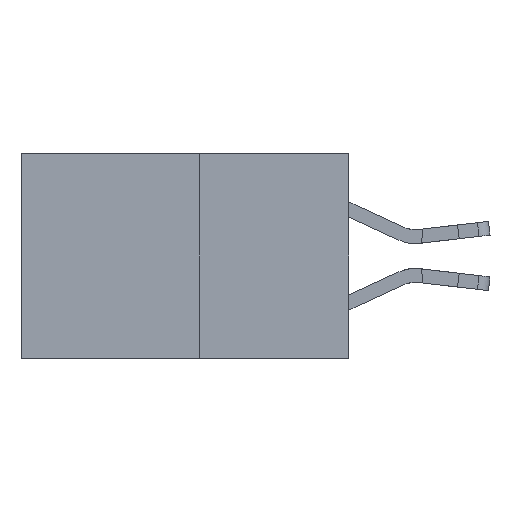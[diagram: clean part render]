
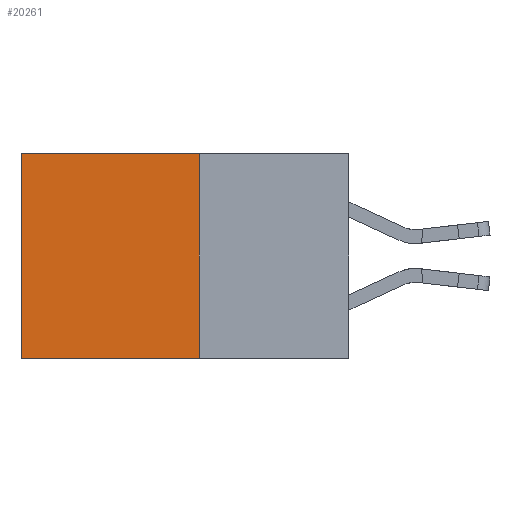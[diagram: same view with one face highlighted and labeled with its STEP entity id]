
A CAD part, left-side view. The second image highlights one B-rep face of the part: STEP entity #20261.
In plain terms, the highlighted planar face has unit normal (-1, 0, 0).
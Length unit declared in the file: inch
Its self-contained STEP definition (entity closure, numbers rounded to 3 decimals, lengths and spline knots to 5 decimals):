
#463 = AXIS2_PLACEMENT_3D ( 'NONE', #13396, #16691, #7174 ) ;
#569 = DIRECTION ( 'NONE',  ( 0., 0., -1. ) ) ;
#863 = VECTOR ( 'NONE', #569, 39.37008 ) ;
#1018 = CARTESIAN_POINT ( 'NONE',  ( 0.277, 0.59, 0. ) ) ;
#1181 = CARTESIAN_POINT ( 'NONE',  ( 0.277, 0.59, -0.37 ) ) ;
#1236 = ORIENTED_EDGE ( 'NONE', *, *, #11369, .F. ) ;
#1487 = VERTEX_POINT ( 'NONE', #5907 ) ;
#2316 = PLANE ( 'NONE',  #463 ) ;
#4132 = CARTESIAN_POINT ( 'NONE',  ( 0.277, 0.27, 0. ) ) ;
#5566 = VECTOR ( 'NONE', #6930, 39.37008 ) ;
#5907 = CARTESIAN_POINT ( 'NONE',  ( 0.277, 0.59, -0.37 ) ) ;
#6713 = CARTESIAN_POINT ( 'NONE',  ( 0.277, 0.27, -0.37 ) ) ;
#6930 = DIRECTION ( 'NONE',  ( 0., 0., -1. ) ) ;
#7153 = EDGE_LOOP ( 'NONE', ( #20407, #1236, #18738, #8484 ) ) ;
#7174 = DIRECTION ( 'NONE',  ( 0., 0., -1. ) ) ;
#8484 = ORIENTED_EDGE ( 'NONE', *, *, #11839, .T. ) ;
#8536 = LINE ( 'NONE', #8779, #20174 ) ;
#8779 = CARTESIAN_POINT ( 'NONE',  ( 0.277, 0.27, -0.37 ) ) ;
#10647 = VERTEX_POINT ( 'NONE', #12171 ) ;
#11369 = EDGE_CURVE ( 'NONE', #20252, #1487, #8536, .T. ) ;
#11839 = EDGE_CURVE ( 'NONE', #10647, #14573, #13846, .T. ) ;
#12171 = CARTESIAN_POINT ( 'NONE',  ( 0.277, 0.27, 0. ) ) ;
#12367 = FACE_OUTER_BOUND ( 'NONE', #7153, .T. ) ;
#13326 = VECTOR ( 'NONE', #18188, 39.37008 ) ;
#13396 = CARTESIAN_POINT ( 'NONE',  ( 0.277, 0.27, -0.37 ) ) ;
#13846 = LINE ( 'NONE', #4132, #13326 ) ;
#14539 = EDGE_CURVE ( 'NONE', #14573, #1487, #17780, .T. ) ;
#14573 = VERTEX_POINT ( 'NONE', #1018 ) ;
#14833 = EDGE_CURVE ( 'NONE', #10647, #20252, #18753, .T. ) ;
#15022 = CARTESIAN_POINT ( 'NONE',  ( 0.277, 0.27, -0.37 ) ) ;
#16491 = DIRECTION ( 'NONE',  ( 0., 1., 0. ) ) ;
#16691 = DIRECTION ( 'NONE',  ( 1., 0., 0. ) ) ;
#17780 = LINE ( 'NONE', #1181, #863 ) ;
#18188 = DIRECTION ( 'NONE',  ( 0., 1., 0. ) ) ;
#18738 = ORIENTED_EDGE ( 'NONE', *, *, #14833, .F. ) ;
#18753 = LINE ( 'NONE', #6713, #5566 ) ;
#20174 = VECTOR ( 'NONE', #16491, 39.37008 ) ;
#20252 = VERTEX_POINT ( 'NONE', #15022 ) ;
#20261 = ADVANCED_FACE ( 'NONE', ( #12367 ), #2316, .F. ) ;
#20407 = ORIENTED_EDGE ( 'NONE', *, *, #14539, .T. ) ;
